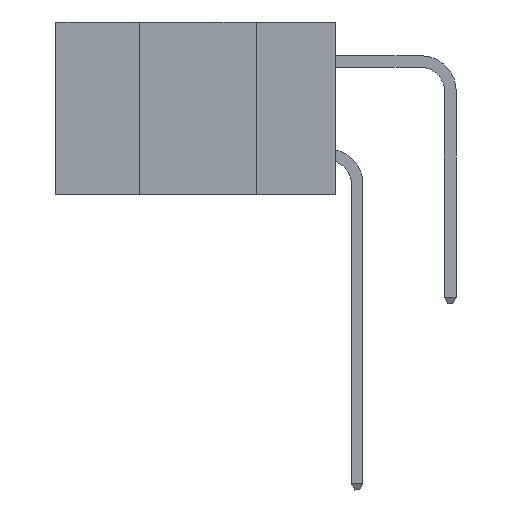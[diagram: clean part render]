
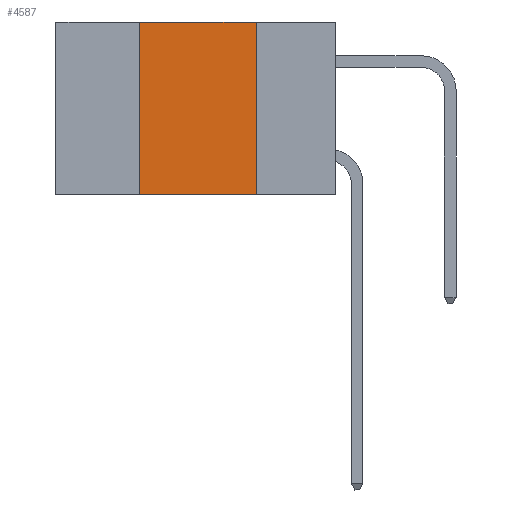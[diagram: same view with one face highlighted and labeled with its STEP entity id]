
A CAD part, left-side view. The second image highlights one B-rep face of the part: STEP entity #4587.
In plain terms, the highlighted planar face has unit normal (-1, 0, 0).
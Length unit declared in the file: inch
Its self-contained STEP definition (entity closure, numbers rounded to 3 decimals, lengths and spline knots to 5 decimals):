
#124 = DIRECTION ( 'NONE',  ( 0., -1., 0. ) ) ;
#1610 = ORIENTED_EDGE ( 'NONE', *, *, #18275, .F. ) ;
#2123 = VECTOR ( 'NONE', #19777, 39.37008 ) ;
#2159 = VERTEX_POINT ( 'NONE', #13367 ) ;
#2871 = CARTESIAN_POINT ( 'NONE',  ( 0., 0.42, -0.37 ) ) ;
#3411 = EDGE_CURVE ( 'NONE', #31660, #25352, #30494, .T. ) ;
#4016 = CARTESIAN_POINT ( 'NONE',  ( 0., 0.42, 0. ) ) ;
#4073 = CARTESIAN_POINT ( 'NONE',  ( 0., 0.17, 0. ) ) ;
#4163 = VERTEX_POINT ( 'NONE', #2871 ) ;
#4587 = ADVANCED_FACE ( 'NONE', ( #11819 ), #4594, .F. ) ;
#4594 = PLANE ( 'NONE',  #15101 ) ;
#5715 = CARTESIAN_POINT ( 'NONE',  ( 0., 0.6, 0. ) ) ;
#6966 = CARTESIAN_POINT ( 'NONE',  ( 0., 0.6, -0.37 ) ) ;
#11819 = FACE_OUTER_BOUND ( 'NONE', #44718, .T. ) ;
#13367 = CARTESIAN_POINT ( 'NONE',  ( 0., 0.17, -0.37 ) ) ;
#14673 = DIRECTION ( 'NONE',  ( 0., 0., -1. ) ) ;
#14891 = ORIENTED_EDGE ( 'NONE', *, *, #16812, .T. ) ;
#15048 = VECTOR ( 'NONE', #27605, 39.37008 ) ;
#15101 = AXIS2_PLACEMENT_3D ( 'NONE', #35972, #18656, #14673 ) ;
#16812 = EDGE_CURVE ( 'NONE', #4163, #2159, #26884, .T. ) ;
#18275 = EDGE_CURVE ( 'NONE', #4163, #31660, #35465, .T. ) ;
#18600 = CARTESIAN_POINT ( 'NONE',  ( 0., 0.42, 0. ) ) ;
#18656 = DIRECTION ( 'NONE',  ( 1., 0., 0. ) ) ;
#19777 = DIRECTION ( 'NONE',  ( 0., -1., 0. ) ) ;
#20911 = CARTESIAN_POINT ( 'NONE',  ( 0., 0.17, 0. ) ) ;
#21531 = EDGE_CURVE ( 'NONE', #25352, #2159, #42816, .T. ) ;
#22022 = VECTOR ( 'NONE', #124, 39.37008 ) ;
#22538 = DIRECTION ( 'NONE',  ( 0., 0., 1. ) ) ;
#25352 = VERTEX_POINT ( 'NONE', #4073 ) ;
#25833 = ORIENTED_EDGE ( 'NONE', *, *, #3411, .F. ) ;
#26228 = VECTOR ( 'NONE', #22538, 39.37008 ) ;
#26884 = LINE ( 'NONE', #6966, #22022 ) ;
#27605 = DIRECTION ( 'NONE',  ( 0., 0., -1. ) ) ;
#30494 = LINE ( 'NONE', #5715, #2123 ) ;
#31660 = VERTEX_POINT ( 'NONE', #4016 ) ;
#34621 = ORIENTED_EDGE ( 'NONE', *, *, #21531, .F. ) ;
#35465 = LINE ( 'NONE', #18600, #26228 ) ;
#35972 = CARTESIAN_POINT ( 'NONE',  ( 0., 0.6, 0. ) ) ;
#42816 = LINE ( 'NONE', #20911, #15048 ) ;
#44718 = EDGE_LOOP ( 'NONE', ( #34621, #25833, #1610, #14891 ) ) ;
